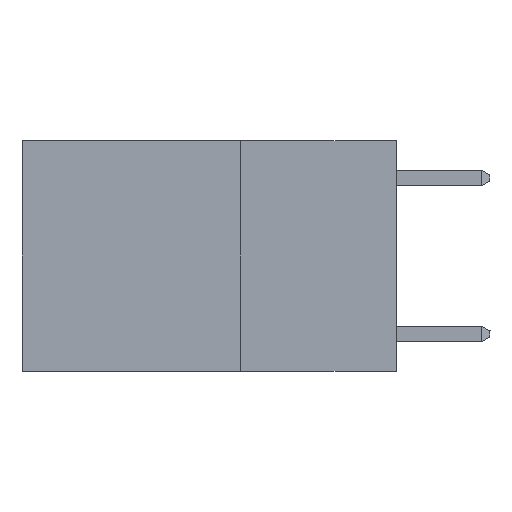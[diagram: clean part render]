
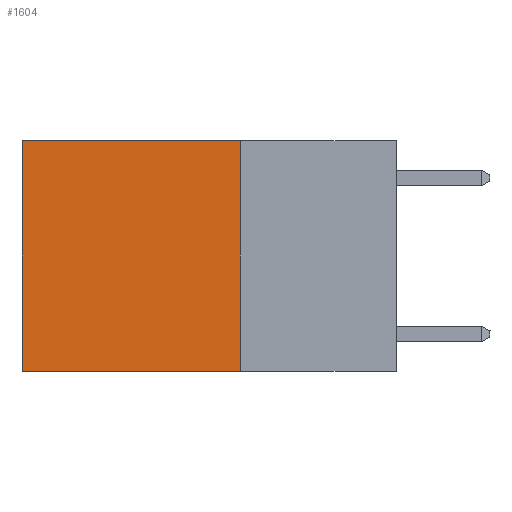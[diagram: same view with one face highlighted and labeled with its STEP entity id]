
A CAD part, left-side view. The second image highlights one B-rep face of the part: STEP entity #1604.
In plain terms, the highlighted planar face has unit normal (-1, 0, 0).
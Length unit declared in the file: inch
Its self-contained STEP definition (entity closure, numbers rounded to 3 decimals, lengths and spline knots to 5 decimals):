
#485 = VECTOR ( 'NONE', #11175, 39.37008 ) ;
#970 = VERTEX_POINT ( 'NONE', #23517 ) ;
#1151 = LINE ( 'NONE', #19088, #485 ) ;
#1604 = ADVANCED_FACE ( 'NONE', ( #14184 ), #25335, .F. ) ;
#1760 = ORIENTED_EDGE ( 'NONE', *, *, #13518, .F. ) ;
#2007 = ORIENTED_EDGE ( 'NONE', *, *, #11837, .T. ) ;
#2583 = CARTESIAN_POINT ( 'NONE',  ( 0.2625, 0.25, 0. ) ) ;
#2675 = DIRECTION ( 'NONE',  ( 0., 1., 0. ) ) ;
#2718 = EDGE_LOOP ( 'NONE', ( #23772, #9395, #1760, #2007 ) ) ;
#3166 = DIRECTION ( 'NONE',  ( 0., 0., -1. ) ) ;
#7520 = VECTOR ( 'NONE', #3166, 39.37008 ) ;
#9395 = ORIENTED_EDGE ( 'NONE', *, *, #22335, .F. ) ;
#9866 = CARTESIAN_POINT ( 'NONE',  ( 0.2625, 0.6, 0. ) ) ;
#11175 = DIRECTION ( 'NONE',  ( 0., 1., 0. ) ) ;
#11607 = CARTESIAN_POINT ( 'NONE',  ( 0.2625, 0.25, 0. ) ) ;
#11670 = LINE ( 'NONE', #9866, #25681 ) ;
#11837 = EDGE_CURVE ( 'NONE', #15603, #17158, #22963, .T. ) ;
#12849 = VERTEX_POINT ( 'NONE', #14178 ) ;
#13518 = EDGE_CURVE ( 'NONE', #15603, #12849, #23162, .T. ) ;
#13628 = CARTESIAN_POINT ( 'NONE',  ( 0.2625, 0.6, 0. ) ) ;
#14178 = CARTESIAN_POINT ( 'NONE',  ( 0.2625, 0.25, -0.37 ) ) ;
#14184 = FACE_OUTER_BOUND ( 'NONE', #2718, .T. ) ;
#15603 = VERTEX_POINT ( 'NONE', #23358 ) ;
#16161 = AXIS2_PLACEMENT_3D ( 'NONE', #25514, #25333, #25272 ) ;
#17158 = VERTEX_POINT ( 'NONE', #13628 ) ;
#17861 = DIRECTION ( 'NONE',  ( 0., 0., -1. ) ) ;
#17885 = EDGE_CURVE ( 'NONE', #17158, #970, #11670, .T. ) ;
#19088 = CARTESIAN_POINT ( 'NONE',  ( 0.2625, 0.25, -0.37 ) ) ;
#21841 = VECTOR ( 'NONE', #2675, 39.37008 ) ;
#22335 = EDGE_CURVE ( 'NONE', #12849, #970, #1151, .T. ) ;
#22963 = LINE ( 'NONE', #2583, #21841 ) ;
#23162 = LINE ( 'NONE', #11607, #7520 ) ;
#23358 = CARTESIAN_POINT ( 'NONE',  ( 0.2625, 0.25, 0. ) ) ;
#23517 = CARTESIAN_POINT ( 'NONE',  ( 0.2625, 0.6, -0.37 ) ) ;
#23772 = ORIENTED_EDGE ( 'NONE', *, *, #17885, .T. ) ;
#25272 = DIRECTION ( 'NONE',  ( 0., 0., -1. ) ) ;
#25333 = DIRECTION ( 'NONE',  ( 1., 0., 0. ) ) ;
#25335 = PLANE ( 'NONE',  #16161 ) ;
#25514 = CARTESIAN_POINT ( 'NONE',  ( 0.2625, 0.25, 0. ) ) ;
#25681 = VECTOR ( 'NONE', #17861, 39.37008 ) ;
